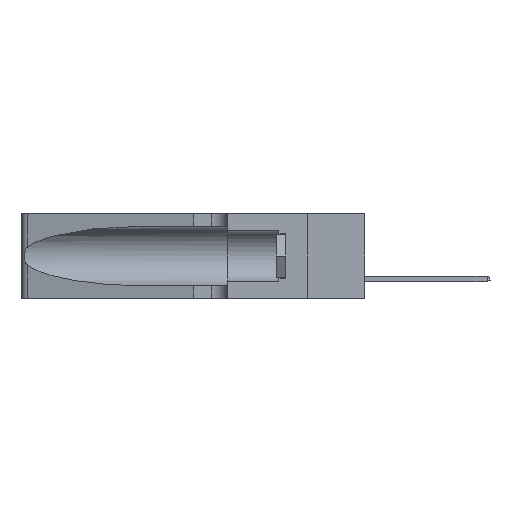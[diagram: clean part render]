
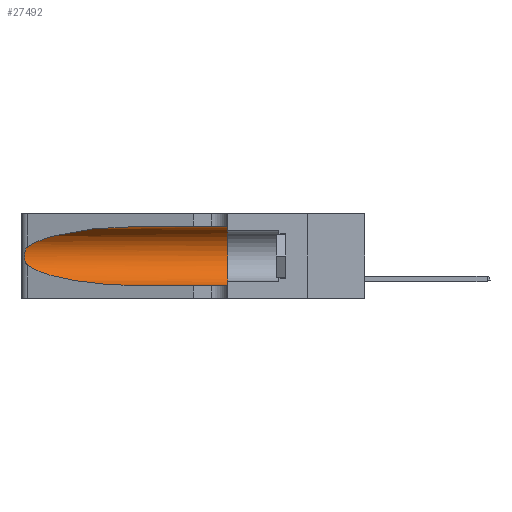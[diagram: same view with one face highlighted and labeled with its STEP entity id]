
A CAD part, left-side view. The second image highlights one B-rep face of the part: STEP entity #27492.
In plain terms, the highlighted cylindrical face has radius 3.308 mm (diameter 6.617 mm), a partial arc.
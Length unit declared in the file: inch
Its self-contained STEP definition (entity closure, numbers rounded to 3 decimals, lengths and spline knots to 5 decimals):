
#271 = CARTESIAN_POINT ( 'NONE',  ( 0.2373, 1.15595, 0.08982 ) ) ;
#342 = CARTESIAN_POINT ( 'NONE',  ( 0.25789, 1.23486, 0.15765 ) ) ;
#424 = CARTESIAN_POINT ( 'NONE',  ( 0.1305, 1.61858, 0.185 ) ) ;
#992 = ORIENTED_EDGE ( 'NONE', *, *, #21228, .F. ) ;
#1922 = VERTEX_POINT ( 'NONE', #33413 ) ;
#2025 = AXIS2_PLACEMENT_3D ( 'NONE', #29823, #29926, #10717 ) ;
#3111 = ORIENTED_EDGE ( 'NONE', *, *, #24286, .T. ) ;
#4985 = VERTEX_POINT ( 'NONE', #26442 ) ;
#5510 = CARTESIAN_POINT ( 'NONE',  ( 0.1305, 0.72297, 0.05475 ) ) ;
#5784 = CARTESIAN_POINT ( 'NONE',  ( 0.25787, 1.23484, 0.2124 ) ) ;
#6635 = VERTEX_POINT ( 'NONE', #13522 ) ;
#6828 = VERTEX_POINT ( 'NONE', #28496 ) ;
#7158 = CARTESIAN_POINT ( 'NONE',  ( 0.1305, 1.61858, 0.31525 ) ) ;
#7170 = LINE ( 'NONE', #27380, #35524 ) ;
#8370 = CARTESIAN_POINT ( 'NONE',  ( 0.25487, 1.22718, 0.14631 ) ) ;
#9525 = EDGE_CURVE ( 'NONE', #1922, #10990, #10215, .T. ) ;
#10215 = CIRCLE ( 'NONE', #2025, 0.13025 ) ;
#10717 = DIRECTION ( 'NONE',  ( 0., 0., 1. ) ) ;
#10990 = VERTEX_POINT ( 'NONE', #14535 ) ;
#11227 = CARTESIAN_POINT ( 'NONE',  ( 0.25639, 1.23184, 0.21858 ) ) ;
#11277 = DIRECTION ( 'NONE',  ( 0., -1., 0. ) ) ;
#12358 = EDGE_CURVE ( 'NONE', #6828, #4985, #33497, .T. ) ;
#12607 = CARTESIAN_POINT ( 'NONE',  ( 0.2373, 1.15595, 0.28018 ) ) ;
#13522 = CARTESIAN_POINT ( 'NONE',  ( 0.1305, 0.72297, 0.05475 ) ) ;
#13961 = ORIENTED_EDGE ( 'NONE', *, *, #21974, .T. ) ;
#14460 = CARTESIAN_POINT ( 'NONE',  ( 0.25856, 1.23593, 0.16098 ) ) ;
#14470 = EDGE_CURVE ( 'NONE', #6635, #10990, #7170, .T. ) ;
#14535 = CARTESIAN_POINT ( 'NONE',  ( 0.1305, 0.35, 0.05475 ) ) ;
#16708 = DIRECTION ( 'NONE',  ( 0., 0., -1. ) ) ;
#16967 = B_SPLINE_CURVE_WITH_KNOTS ( 'NONE', 3,
 ( #33212, #33569, #11227, #5784, #25258, #30783, #33315, #30428, #27890, #14460, #342, #19987, #25019, #19646 ),
 .UNSPECIFIED., .F., .F.,
 ( 4, 2, 2, 2, 2, 2, 4 ),
 ( 0., 0.00027, 0.00053, 0.00107, 0.0016, 0.00187, 0.00214 ),
 .UNSPECIFIED. ) ;
#17545 = LINE ( 'NONE', #7158, #18859 ) ;
#17976 = CARTESIAN_POINT ( 'NONE',  ( 0.1305, 0.72297, 0.31525 ) ) ;
#18137 = AXIS2_PLACEMENT_3D ( 'NONE', #424, #19260, #16708 ) ;
#18859 = VECTOR ( 'NONE', #20888, 39.37008 ) ;
#19127 = FACE_OUTER_BOUND ( 'NONE', #31682, .T. ) ;
#19260 = DIRECTION ( 'NONE',  ( 0., -1., 0. ) ) ;
#19578 = CARTESIAN_POINT ( 'NONE',  ( 0.18966, 0.96281, 0.05475 ) ) ;
#19646 = CARTESIAN_POINT ( 'NONE',  ( 0.25487, 1.22718, 0.14631 ) ) ;
#19987 = CARTESIAN_POINT ( 'NONE',  ( 0.25639, 1.23186, 0.15144 ) ) ;
#20258 = CARTESIAN_POINT ( 'NONE',  ( 0.25487, 1.22718, 0.14631 ) ) ;
#20888 = DIRECTION ( 'NONE',  ( 0., -1., 0. ) ) ;
#21060 = VERTEX_POINT ( 'NONE', #20258 ) ;
#21228 = EDGE_CURVE ( 'NONE', #6828, #1922, #17545, .T. ) ;
#21974 = EDGE_CURVE ( 'NONE', #4985, #21060, #16967, .T. ) ;
#23378 = CARTESIAN_POINT ( 'NONE',  ( 0.18966, 0.96281, 0.31525 ) ) ;
#24286 = EDGE_CURVE ( 'NONE', #21060, #6635, #26047, .T. ) ;
#25019 = CARTESIAN_POINT ( 'NONE',  ( 0.25555, 1.22993, 0.14849 ) ) ;
#25258 = CARTESIAN_POINT ( 'NONE',  ( 0.25854, 1.2359, 0.20912 ) ) ;
#26047 =( BOUNDED_CURVE ( )  B_SPLINE_CURVE ( 3, ( #8370, #271, #19578, #5510 ),
 .UNSPECIFIED., .F., .F. ) 
 B_SPLINE_CURVE_WITH_KNOTS ( ( 4, 4 ),
 ( 3.44316, 4.71239 ),
 .UNSPECIFIED. ) 
 CURVE ( )  GEOMETRIC_REPRESENTATION_ITEM ( )  RATIONAL_B_SPLINE_CURVE ( ( 1., 0.87, 0.87, 1. ) ) 
 REPRESENTATION_ITEM ( '' )  );
#26442 = CARTESIAN_POINT ( 'NONE',  ( 0.25487, 1.22718, 0.22369 ) ) ;
#26514 = ORIENTED_EDGE ( 'NONE', *, *, #14470, .T. ) ;
#27380 = CARTESIAN_POINT ( 'NONE',  ( 0.1305, 1.61858, 0.05475 ) ) ;
#27492 = ADVANCED_FACE ( 'NONE', ( #19127 ), #29870, .F. ) ;
#27496 = ORIENTED_EDGE ( 'NONE', *, *, #12358, .T. ) ;
#27890 = CARTESIAN_POINT ( 'NONE',  ( 0.26017, 1.23833, 0.17102 ) ) ;
#28496 = CARTESIAN_POINT ( 'NONE',  ( 0.1305, 0.72297, 0.31525 ) ) ;
#29823 = CARTESIAN_POINT ( 'NONE',  ( 0.1305, 0.35, 0.185 ) ) ;
#29870 = CYLINDRICAL_SURFACE ( 'NONE', #18137, 0.13025 ) ;
#29926 = DIRECTION ( 'NONE',  ( 0., 1., 0. ) ) ;
#30428 = CARTESIAN_POINT ( 'NONE',  ( 0.26075, 1.23896, 0.178 ) ) ;
#30783 = CARTESIAN_POINT ( 'NONE',  ( 0.26018, 1.23835, 0.19895 ) ) ;
#31307 = CARTESIAN_POINT ( 'NONE',  ( 0.25487, 1.22718, 0.22369 ) ) ;
#31682 = EDGE_LOOP ( 'NONE', ( #27496, #13961, #3111, #26514, #32128, #992 ) ) ;
#32128 = ORIENTED_EDGE ( 'NONE', *, *, #9525, .F. ) ;
#33212 = CARTESIAN_POINT ( 'NONE',  ( 0.25487, 1.22718, 0.22369 ) ) ;
#33315 = CARTESIAN_POINT ( 'NONE',  ( 0.26075, 1.23896, 0.19203 ) ) ;
#33413 = CARTESIAN_POINT ( 'NONE',  ( 0.1305, 0.35, 0.31525 ) ) ;
#33497 =( BOUNDED_CURVE ( )  B_SPLINE_CURVE ( 3, ( #17976, #23378, #12607, #31307 ),
 .UNSPECIFIED., .F., .F. ) 
 B_SPLINE_CURVE_WITH_KNOTS ( ( 4, 4 ),
 ( 1.5708, 2.84003 ),
 .UNSPECIFIED. ) 
 CURVE ( )  GEOMETRIC_REPRESENTATION_ITEM ( )  RATIONAL_B_SPLINE_CURVE ( ( 1., 0.87, 0.87, 1. ) ) 
 REPRESENTATION_ITEM ( '' )  );
#33569 = CARTESIAN_POINT ( 'NONE',  ( 0.25555, 1.22994, 0.2215 ) ) ;
#35524 = VECTOR ( 'NONE', #11277, 39.37008 ) ;
